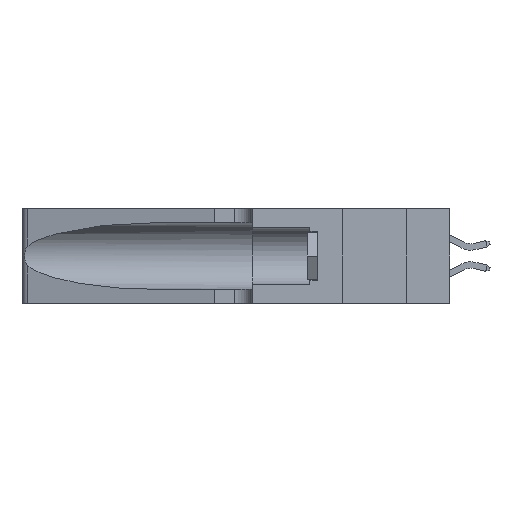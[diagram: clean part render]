
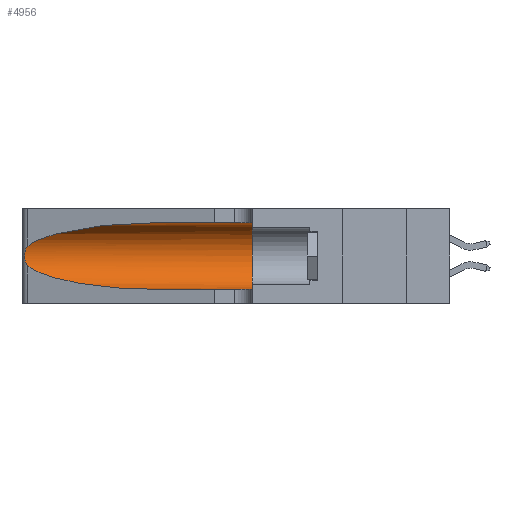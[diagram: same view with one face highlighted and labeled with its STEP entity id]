
A CAD part, left-side view. The second image highlights one B-rep face of the part: STEP entity #4956.
In plain terms, the highlighted cylindrical face has radius 3.308 mm (diameter 6.617 mm), a partial arc.
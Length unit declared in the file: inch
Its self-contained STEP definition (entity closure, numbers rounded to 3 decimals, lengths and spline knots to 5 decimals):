
#456 = CARTESIAN_POINT ( 'NONE',  ( 0.26017, 1.23833, 0.17102 ) ) ;
#850 = EDGE_CURVE ( 'NONE', #19202, #8163, #18040, .T. ) ;
#1430 = DIRECTION ( 'NONE',  ( 0., -1., 0. ) ) ;
#1533 = EDGE_CURVE ( 'NONE', #21340, #15632, #11680, .T. ) ;
#3016 = CARTESIAN_POINT ( 'NONE',  ( 0.25789, 1.23486, 0.15765 ) ) ;
#3475 = CARTESIAN_POINT ( 'NONE',  ( 0.25555, 1.22993, 0.14849 ) ) ;
#4128 = EDGE_CURVE ( 'NONE', #17181, #21340, #29703, .T. ) ;
#4956 = ADVANCED_FACE ( 'NONE', ( #13877 ), #27160, .F. ) ;
#5414 = CARTESIAN_POINT ( 'NONE',  ( 0.26075, 1.23896, 0.19203 ) ) ;
#6410 = EDGE_LOOP ( 'NONE', ( #22687, #20354, #29957, #20325, #25806, #35188 ) ) ;
#6498 = CARTESIAN_POINT ( 'NONE',  ( 0.25487, 1.22718, 0.22369 ) ) ;
#6577 = CARTESIAN_POINT ( 'NONE',  ( 0.18966, 0.96281, 0.05475 ) ) ;
#6651 = EDGE_CURVE ( 'NONE', #15632, #33066, #22068, .T. ) ;
#7721 = CARTESIAN_POINT ( 'NONE',  ( 0.1305, 0.72297, 0.31525 ) ) ;
#8163 = VERTEX_POINT ( 'NONE', #11669 ) ;
#8680 = CARTESIAN_POINT ( 'NONE',  ( 0.25856, 1.23593, 0.16098 ) ) ;
#9640 = DIRECTION ( 'NONE',  ( 0., -1., 0. ) ) ;
#10420 = AXIS2_PLACEMENT_3D ( 'NONE', #12646, #17592, #25944 ) ;
#10772 = CARTESIAN_POINT ( 'NONE',  ( 0.25854, 1.2359, 0.20912 ) ) ;
#11116 = CARTESIAN_POINT ( 'NONE',  ( 0.25555, 1.22994, 0.2215 ) ) ;
#11669 = CARTESIAN_POINT ( 'NONE',  ( 0.1305, 0.35, 0.31525 ) ) ;
#11680 =( BOUNDED_CURVE ( )  B_SPLINE_CURVE ( 3, ( #14704, #20142, #6577, #17751 ),
 .UNSPECIFIED., .F., .F. ) 
 B_SPLINE_CURVE_WITH_KNOTS ( ( 4, 4 ),
 ( 3.44316, 4.71239 ),
 .UNSPECIFIED. ) 
 CURVE ( )  GEOMETRIC_REPRESENTATION_ITEM ( )  RATIONAL_B_SPLINE_CURVE ( ( 1., 0.87, 0.87, 1. ) ) 
 REPRESENTATION_ITEM ( '' )  );
#12646 = CARTESIAN_POINT ( 'NONE',  ( 0.1305, 0.35, 0.185 ) ) ;
#13404 = CARTESIAN_POINT ( 'NONE',  ( 0.26018, 1.23835, 0.19895 ) ) ;
#13462 =( BOUNDED_CURVE ( )  B_SPLINE_CURVE ( 3, ( #16885, #28167, #27933, #14535 ),
 .UNSPECIFIED., .F., .T. ) 
 B_SPLINE_CURVE_WITH_KNOTS ( ( 4, 4 ),
 ( 1.5708, 2.84003 ),
 .UNSPECIFIED. ) 
 CURVE ( )  GEOMETRIC_REPRESENTATION_ITEM ( )  RATIONAL_B_SPLINE_CURVE ( ( 1., 0.87, 0.87, 1. ) ) 
 REPRESENTATION_ITEM ( '' )  );
#13877 = FACE_OUTER_BOUND ( 'NONE', #6410, .T. ) ;
#14535 = CARTESIAN_POINT ( 'NONE',  ( 0.25487, 1.22718, 0.22369 ) ) ;
#14704 = CARTESIAN_POINT ( 'NONE',  ( 0.25487, 1.22718, 0.14631 ) ) ;
#14901 = CARTESIAN_POINT ( 'NONE',  ( 0.1305, 1.61858, 0.185 ) ) ;
#15632 = VERTEX_POINT ( 'NONE', #23270 ) ;
#15735 = CARTESIAN_POINT ( 'NONE',  ( 0.1305, 0.35, 0.05475 ) ) ;
#16132 = CARTESIAN_POINT ( 'NONE',  ( 0.1305, 1.61858, 0.05475 ) ) ;
#16148 = VECTOR ( 'NONE', #21799, 39.37008 ) ;
#16326 = VECTOR ( 'NONE', #9640, 39.37008 ) ;
#16885 = CARTESIAN_POINT ( 'NONE',  ( 0.1305, 0.72297, 0.31525 ) ) ;
#17181 = VERTEX_POINT ( 'NONE', #6498 ) ;
#17592 = DIRECTION ( 'NONE',  ( 0., 1., 0. ) ) ;
#17751 = CARTESIAN_POINT ( 'NONE',  ( 0.1305, 0.72297, 0.05475 ) ) ;
#18040 = LINE ( 'NONE', #29241, #16326 ) ;
#19202 = VERTEX_POINT ( 'NONE', #7721 ) ;
#20142 = CARTESIAN_POINT ( 'NONE',  ( 0.2373, 1.15595, 0.08982 ) ) ;
#20325 = ORIENTED_EDGE ( 'NONE', *, *, #6651, .T. ) ;
#20354 = ORIENTED_EDGE ( 'NONE', *, *, #4128, .T. ) ;
#21340 = VERTEX_POINT ( 'NONE', #33454 ) ;
#21799 = DIRECTION ( 'NONE',  ( 0., -1., 0. ) ) ;
#22068 = LINE ( 'NONE', #16132, #16148 ) ;
#22515 = CARTESIAN_POINT ( 'NONE',  ( 0.26075, 1.23896, 0.178 ) ) ;
#22687 = ORIENTED_EDGE ( 'NONE', *, *, #34952, .T. ) ;
#23270 = CARTESIAN_POINT ( 'NONE',  ( 0.1305, 0.72297, 0.05475 ) ) ;
#24902 = CARTESIAN_POINT ( 'NONE',  ( 0.25487, 1.22718, 0.14631 ) ) ;
#25235 = CARTESIAN_POINT ( 'NONE',  ( 0.25639, 1.23186, 0.15144 ) ) ;
#25806 = ORIENTED_EDGE ( 'NONE', *, *, #29490, .F. ) ;
#25944 = DIRECTION ( 'NONE',  ( 0., 0., 1. ) ) ;
#26076 = DIRECTION ( 'NONE',  ( 0., 0., -1. ) ) ;
#27037 = CARTESIAN_POINT ( 'NONE',  ( 0.25487, 1.22718, 0.22369 ) ) ;
#27160 = CYLINDRICAL_SURFACE ( 'NONE', #33471, 0.13025 ) ;
#27933 = CARTESIAN_POINT ( 'NONE',  ( 0.2373, 1.15595, 0.28018 ) ) ;
#28167 = CARTESIAN_POINT ( 'NONE',  ( 0.18966, 0.96281, 0.31525 ) ) ;
#28472 = CIRCLE ( 'NONE', #10420, 0.13025 ) ;
#29241 = CARTESIAN_POINT ( 'NONE',  ( 0.1305, 1.61858, 0.31525 ) ) ;
#29490 = EDGE_CURVE ( 'NONE', #8163, #33066, #28472, .T. ) ;
#29703 = B_SPLINE_CURVE_WITH_KNOTS ( 'NONE', 3,
 ( #27037, #11116, #30267, #29805, #10772, #13404, #5414, #22515, #456, #8680, #3016, #25235, #3475, #24902 ),
 .UNSPECIFIED., .F., .F.,
 ( 4, 2, 2, 2, 2, 2, 4 ),
 ( 0., 0.00027, 0.00053, 0.00107, 0.0016, 0.00187, 0.00214 ),
 .UNSPECIFIED. ) ;
#29805 = CARTESIAN_POINT ( 'NONE',  ( 0.25787, 1.23484, 0.2124 ) ) ;
#29957 = ORIENTED_EDGE ( 'NONE', *, *, #1533, .T. ) ;
#30267 = CARTESIAN_POINT ( 'NONE',  ( 0.25639, 1.23184, 0.21858 ) ) ;
#33066 = VERTEX_POINT ( 'NONE', #15735 ) ;
#33454 = CARTESIAN_POINT ( 'NONE',  ( 0.25487, 1.22718, 0.14631 ) ) ;
#33471 = AXIS2_PLACEMENT_3D ( 'NONE', #14901, #1430, #26076 ) ;
#34952 = EDGE_CURVE ( 'NONE', #19202, #17181, #13462, .T. ) ;
#35188 = ORIENTED_EDGE ( 'NONE', *, *, #850, .F. ) ;
